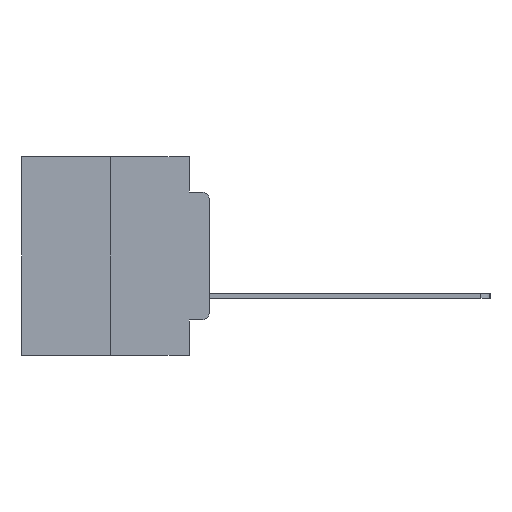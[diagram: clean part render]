
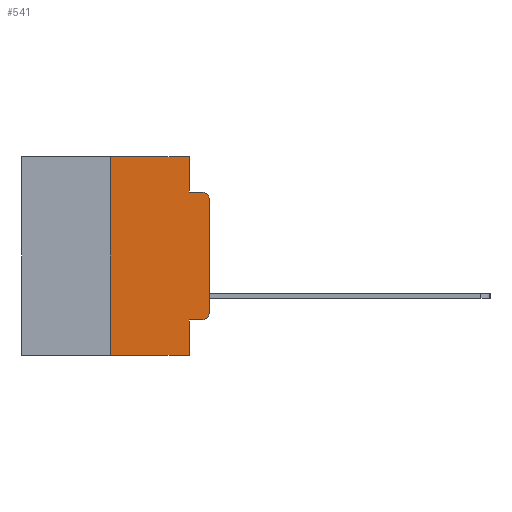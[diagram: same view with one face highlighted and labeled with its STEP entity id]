
A CAD part, left-side view. The second image highlights one B-rep face of the part: STEP entity #541.
In plain terms, the highlighted planar face has unit normal (-1, 0, 0).
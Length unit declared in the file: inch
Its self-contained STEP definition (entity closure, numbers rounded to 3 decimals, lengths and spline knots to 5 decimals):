
#520 = LINE ( 'NONE', #2200, #11283 ) ;
#541 = ADVANCED_FACE ( 'NONE', ( #22766 ), #7877, .F. ) ;
#690 = EDGE_CURVE ( 'NONE', #22329, #9295, #15375, .T. ) ;
#885 = CARTESIAN_POINT ( 'NONE',  ( 0., 0.051, -0.4115 ) ) ;
#902 = CARTESIAN_POINT ( 'NONE',  ( 0., 0.02, -0.1085 ) ) ;
#948 = LINE ( 'NONE', #8896, #21907 ) ;
#1277 = AXIS2_PLACEMENT_3D ( 'NONE', #14520, #14362, #25203 ) ;
#2134 = VERTEX_POINT ( 'NONE', #8386 ) ;
#2200 = CARTESIAN_POINT ( 'NONE',  ( 0., 0.051, -0.0885 ) ) ;
#2319 = VERTEX_POINT ( 'NONE', #19389 ) ;
#2639 = EDGE_CURVE ( 'NONE', #9032, #11550, #20379, .T. ) ;
#3004 = EDGE_CURVE ( 'NONE', #2134, #2319, #14100, .T. ) ;
#4462 = EDGE_CURVE ( 'NONE', #11550, #2134, #14424, .T. ) ;
#4489 = CARTESIAN_POINT ( 'NONE',  ( 0., 0.25, 0. ) ) ;
#4796 = ORIENTED_EDGE ( 'NONE', *, *, #4462, .T. ) ;
#5105 = AXIS2_PLACEMENT_3D ( 'NONE', #902, #10437, #6257 ) ;
#6078 = CARTESIAN_POINT ( 'NONE',  ( 0., 0.473, 0. ) ) ;
#6163 = EDGE_LOOP ( 'NONE', ( #4796, #20872, #25736, #11826, #22607, #13073, #19449, #20025, #24855, #10265 ) ) ;
#6257 = DIRECTION ( 'NONE',  ( 0., 0., -1. ) ) ;
#7877 = PLANE ( 'NONE',  #1277 ) ;
#8337 = CARTESIAN_POINT ( 'NONE',  ( 0., 0.051, 0. ) ) ;
#8386 = CARTESIAN_POINT ( 'NONE',  ( 0., 0., -0.1085 ) ) ;
#8896 = CARTESIAN_POINT ( 'NONE',  ( 0., 0.473, -0.5 ) ) ;
#9032 = VERTEX_POINT ( 'NONE', #22699 ) ;
#9057 = VECTOR ( 'NONE', #10579, 39.37008 ) ;
#9152 = VERTEX_POINT ( 'NONE', #19631 ) ;
#9295 = VERTEX_POINT ( 'NONE', #18381 ) ;
#9392 = EDGE_CURVE ( 'NONE', #16526, #9295, #948, .T. ) ;
#9410 = EDGE_CURVE ( 'NONE', #16526, #9152, #16294, .T. ) ;
#10108 = VECTOR ( 'NONE', #14042, 39.37008 ) ;
#10265 = ORIENTED_EDGE ( 'NONE', *, *, #2639, .T. ) ;
#10437 = DIRECTION ( 'NONE',  ( -1., 0., 0. ) ) ;
#10547 = CARTESIAN_POINT ( 'NONE',  ( 0., 0., 0. ) ) ;
#10579 = DIRECTION ( 'NONE',  ( 0., 0., 1. ) ) ;
#10817 = EDGE_CURVE ( 'NONE', #13755, #18751, #11020, .T. ) ;
#10818 = DIRECTION ( 'NONE',  ( 0., -1., 0. ) ) ;
#10936 = CARTESIAN_POINT ( 'NONE',  ( 0., 0.051, 0. ) ) ;
#11020 = LINE ( 'NONE', #8337, #15626 ) ;
#11068 = VECTOR ( 'NONE', #12999, 39.37008 ) ;
#11283 = VECTOR ( 'NONE', #10818, 39.37008 ) ;
#11366 = LINE ( 'NONE', #885, #15988 ) ;
#11550 = VERTEX_POINT ( 'NONE', #18932 ) ;
#11820 = EDGE_CURVE ( 'NONE', #9152, #13755, #13135, .T. ) ;
#11826 = ORIENTED_EDGE ( 'NONE', *, *, #10817, .F. ) ;
#11898 = CARTESIAN_POINT ( 'NONE',  ( 0., 0.25, -0.5 ) ) ;
#12741 = AXIS2_PLACEMENT_3D ( 'NONE', #16928, #13711, #15088 ) ;
#12999 = DIRECTION ( 'NONE',  ( 0., 0., 1. ) ) ;
#13073 = ORIENTED_EDGE ( 'NONE', *, *, #9410, .F. ) ;
#13135 = LINE ( 'NONE', #6078, #22654 ) ;
#13711 = DIRECTION ( 'NONE',  ( -1., 0., 0. ) ) ;
#13755 = VERTEX_POINT ( 'NONE', #10936 ) ;
#14042 = DIRECTION ( 'NONE',  ( 0., 0., -1. ) ) ;
#14100 = CIRCLE ( 'NONE', #5105, 0.02 ) ;
#14362 = DIRECTION ( 'NONE',  ( 1., 0., 0. ) ) ;
#14424 = LINE ( 'NONE', #10547, #9057 ) ;
#14520 = CARTESIAN_POINT ( 'NONE',  ( 0., 0.473, 0. ) ) ;
#15088 = DIRECTION ( 'NONE',  ( 0., 0., -1. ) ) ;
#15375 = LINE ( 'NONE', #23842, #10108 ) ;
#15626 = VECTOR ( 'NONE', #22026, 39.37008 ) ;
#15988 = VECTOR ( 'NONE', #17455, 39.37008 ) ;
#16294 = LINE ( 'NONE', #4489, #11068 ) ;
#16526 = VERTEX_POINT ( 'NONE', #11898 ) ;
#16928 = CARTESIAN_POINT ( 'NONE',  ( 0., 0.02, -0.3915 ) ) ;
#17455 = DIRECTION ( 'NONE',  ( 0., -1., 0. ) ) ;
#18381 = CARTESIAN_POINT ( 'NONE',  ( 0., 0.051, -0.5 ) ) ;
#18445 = CARTESIAN_POINT ( 'NONE',  ( 0., 0.051, -0.4115 ) ) ;
#18751 = VERTEX_POINT ( 'NONE', #25259 ) ;
#18932 = CARTESIAN_POINT ( 'NONE',  ( 0., 0., -0.3915 ) ) ;
#19389 = CARTESIAN_POINT ( 'NONE',  ( 0., 0.02, -0.0885 ) ) ;
#19449 = ORIENTED_EDGE ( 'NONE', *, *, #9392, .T. ) ;
#19631 = CARTESIAN_POINT ( 'NONE',  ( 0., 0.25, 0. ) ) ;
#20025 = ORIENTED_EDGE ( 'NONE', *, *, #690, .F. ) ;
#20379 = CIRCLE ( 'NONE', #12741, 0.02 ) ;
#20407 = EDGE_CURVE ( 'NONE', #22329, #9032, #11366, .T. ) ;
#20872 = ORIENTED_EDGE ( 'NONE', *, *, #3004, .T. ) ;
#21907 = VECTOR ( 'NONE', #22501, 39.37008 ) ;
#21987 = DIRECTION ( 'NONE',  ( 0., -1., 0. ) ) ;
#22026 = DIRECTION ( 'NONE',  ( 0., 0., -1. ) ) ;
#22329 = VERTEX_POINT ( 'NONE', #18445 ) ;
#22406 = EDGE_CURVE ( 'NONE', #18751, #2319, #520, .T. ) ;
#22501 = DIRECTION ( 'NONE',  ( 0., -1., 0. ) ) ;
#22607 = ORIENTED_EDGE ( 'NONE', *, *, #11820, .F. ) ;
#22654 = VECTOR ( 'NONE', #21987, 39.37008 ) ;
#22699 = CARTESIAN_POINT ( 'NONE',  ( 0., 0.02, -0.4115 ) ) ;
#22766 = FACE_OUTER_BOUND ( 'NONE', #6163, .T. ) ;
#23842 = CARTESIAN_POINT ( 'NONE',  ( 0., 0.051, 0. ) ) ;
#24855 = ORIENTED_EDGE ( 'NONE', *, *, #20407, .T. ) ;
#25203 = DIRECTION ( 'NONE',  ( 0., 0., -1. ) ) ;
#25259 = CARTESIAN_POINT ( 'NONE',  ( 0., 0.051, -0.0885 ) ) ;
#25736 = ORIENTED_EDGE ( 'NONE', *, *, #22406, .F. ) ;
